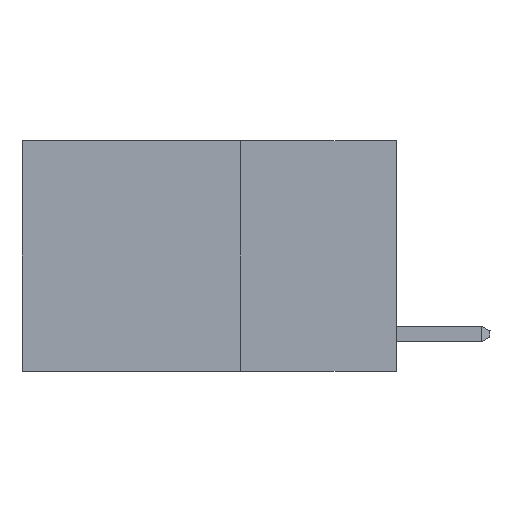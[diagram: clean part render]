
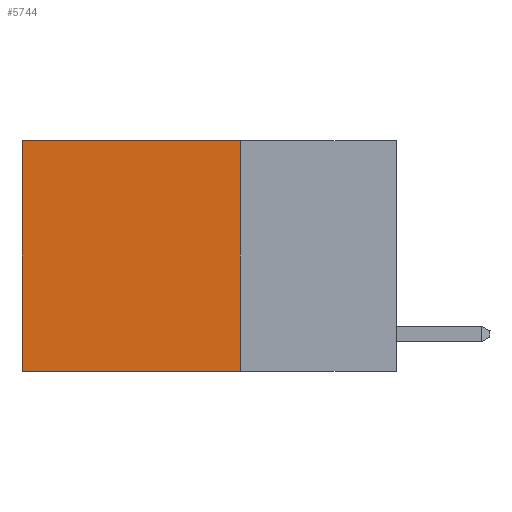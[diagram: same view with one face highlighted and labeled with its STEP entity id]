
A CAD part, left-side view. The second image highlights one B-rep face of the part: STEP entity #5744.
In plain terms, the highlighted planar face has unit normal (-1, 0, 0).
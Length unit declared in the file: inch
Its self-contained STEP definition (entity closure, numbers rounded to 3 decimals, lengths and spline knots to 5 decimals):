
#655 = VECTOR ( 'NONE', #690, 39.37008 ) ;
#690 = DIRECTION ( 'NONE',  ( 0., 1., 0. ) ) ;
#697 = EDGE_LOOP ( 'NONE', ( #7585, #1556, #8672, #9237 ) ) ;
#767 = CARTESIAN_POINT ( 'NONE',  ( 0.2625, 0.6, 0. ) ) ;
#955 = DIRECTION ( 'NONE',  ( 0., 0., -1. ) ) ;
#1457 = VERTEX_POINT ( 'NONE', #8241 ) ;
#1556 = ORIENTED_EDGE ( 'NONE', *, *, #4527, .F. ) ;
#1929 = LINE ( 'NONE', #8900, #11103 ) ;
#2378 = EDGE_CURVE ( 'NONE', #1457, #10488, #11396, .T. ) ;
#3505 = PLANE ( 'NONE',  #7561 ) ;
#4127 = VECTOR ( 'NONE', #10758, 39.37008 ) ;
#4372 = EDGE_CURVE ( 'NONE', #10264, #4965, #7092, .T. ) ;
#4527 = EDGE_CURVE ( 'NONE', #4965, #10488, #6557, .T. ) ;
#4965 = VERTEX_POINT ( 'NONE', #6506 ) ;
#5465 = VECTOR ( 'NONE', #955, 39.37008 ) ;
#5744 = ADVANCED_FACE ( 'NONE', ( #6307 ), #3505, .F. ) ;
#5966 = EDGE_CURVE ( 'NONE', #10264, #1457, #1929, .T. ) ;
#6307 = FACE_OUTER_BOUND ( 'NONE', #697, .T. ) ;
#6312 = CARTESIAN_POINT ( 'NONE',  ( 0.2625, 0.25, 0. ) ) ;
#6506 = CARTESIAN_POINT ( 'NONE',  ( 0.2625, 0.25, -0.37 ) ) ;
#6557 = LINE ( 'NONE', #9667, #655 ) ;
#6768 = DIRECTION ( 'NONE',  ( 1., 0., 0. ) ) ;
#7092 = LINE ( 'NONE', #6312, #4127 ) ;
#7424 = DIRECTION ( 'NONE',  ( 0., 0., -1. ) ) ;
#7561 = AXIS2_PLACEMENT_3D ( 'NONE', #9135, #6768, #7424 ) ;
#7585 = ORIENTED_EDGE ( 'NONE', *, *, #2378, .T. ) ;
#8185 = DIRECTION ( 'NONE',  ( 0., 1., 0. ) ) ;
#8241 = CARTESIAN_POINT ( 'NONE',  ( 0.2625, 0.6, 0. ) ) ;
#8672 = ORIENTED_EDGE ( 'NONE', *, *, #4372, .F. ) ;
#8900 = CARTESIAN_POINT ( 'NONE',  ( 0.2625, 0.25, 0. ) ) ;
#9135 = CARTESIAN_POINT ( 'NONE',  ( 0.2625, 0.25, 0. ) ) ;
#9237 = ORIENTED_EDGE ( 'NONE', *, *, #5966, .T. ) ;
#9667 = CARTESIAN_POINT ( 'NONE',  ( 0.2625, 0.25, -0.37 ) ) ;
#9688 = CARTESIAN_POINT ( 'NONE',  ( 0.2625, 0.25, 0. ) ) ;
#10264 = VERTEX_POINT ( 'NONE', #9688 ) ;
#10380 = CARTESIAN_POINT ( 'NONE',  ( 0.2625, 0.6, -0.37 ) ) ;
#10488 = VERTEX_POINT ( 'NONE', #10380 ) ;
#10758 = DIRECTION ( 'NONE',  ( 0., 0., -1. ) ) ;
#11103 = VECTOR ( 'NONE', #8185, 39.37008 ) ;
#11396 = LINE ( 'NONE', #767, #5465 ) ;
